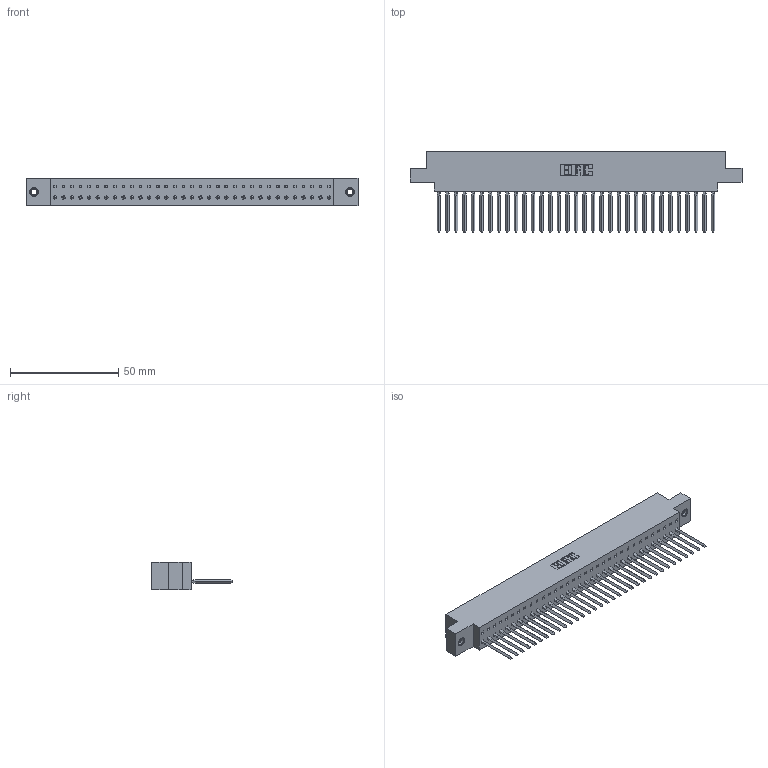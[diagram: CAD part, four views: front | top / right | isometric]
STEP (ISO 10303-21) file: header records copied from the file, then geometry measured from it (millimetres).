
FILE_DESCRIPTION (( 'STEP AP203' ), '1' );
FILE_NAME ('317-033-541-607.STEP', '2020-02-27T21:35:49', ( '' ), ( '' ), 'SwSTEP 2.0', 'SolidWorks 2016', '' );
FILE_SCHEMA (( 'CONFIG_CONTROL_DESIGN' ));
Length unit declared in the file: inch
Products named in the file (4): 317-033-541-607; 317-290-002_541; 317 Part_.156 Dia - TI; 345-250-001_345-250-005-103
Assembly tree (36 placements, depth 2):
  317-033-541-607
    317 Part_.156 Dia - TI
    317-290-002_541  x33
    345-250-001_345-250-005-103  x2
Bounding box: 153.47 x 37.34 x 12.7 mm (x, y, z)
Volume: 24596.9 mm3; surface area: 34492.5 mm2
Topology: 36 solids, 36 shells, 5178 faces, 14733 edges, 9572 vertices
Faces by surface type: plane 4182, cylinder 848, bspline 132, cone 12, torus 4
Entity records: 50635 total; most frequent: CARTESIAN_POINT 9607, ORIENTED_EDGE 8886, DIRECTION 7335, EDGE_CURVE 4443, LINE 4059, VECTOR 4059, VERTEX_POINT 2950, AXIS2_PLACEMENT_3D 1638
